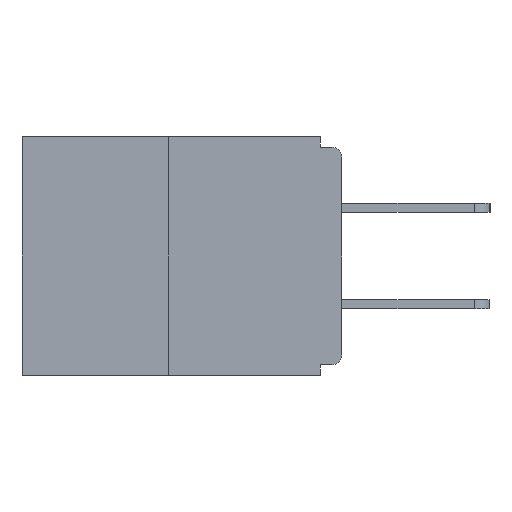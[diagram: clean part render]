
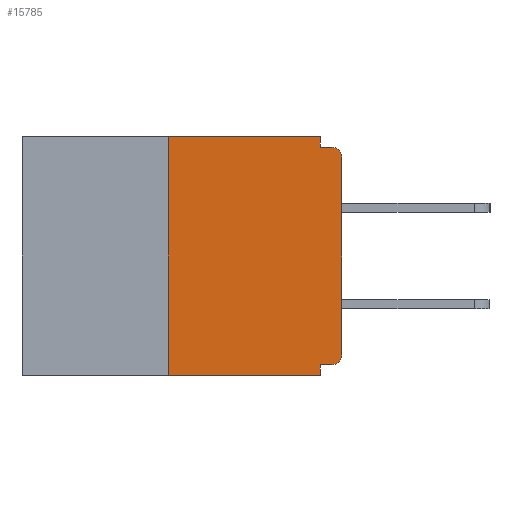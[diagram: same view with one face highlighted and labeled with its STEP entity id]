
A CAD part, left-side view. The second image highlights one B-rep face of the part: STEP entity #15785.
In plain terms, the highlighted planar face has unit normal (-1, 0, 0).
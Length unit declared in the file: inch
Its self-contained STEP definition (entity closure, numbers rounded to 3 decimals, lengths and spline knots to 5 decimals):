
#583 = VERTEX_POINT ( 'NONE', #587 ) ;
#587 = CARTESIAN_POINT ( 'NONE',  ( 0., 0.25, -0.343 ) ) ;
#1026 = ORIENTED_EDGE ( 'NONE', *, *, #21124, .T. ) ;
#1037 = VERTEX_POINT ( 'NONE', #14218 ) ;
#1105 = VECTOR ( 'NONE', #7954, 39.37008 ) ;
#1210 = CARTESIAN_POINT ( 'NONE',  ( 0., 0.031, 0. ) ) ;
#1218 = LINE ( 'NONE', #15127, #15951 ) ;
#1472 = VERTEX_POINT ( 'NONE', #10918 ) ;
#2548 = EDGE_CURVE ( 'NONE', #1472, #4662, #10265, .T. ) ;
#2583 = EDGE_CURVE ( 'NONE', #6001, #6195, #3032, .T. ) ;
#2666 = DIRECTION ( 'NONE',  ( -1., 0., 0. ) ) ;
#2923 = DIRECTION ( 'NONE',  ( 0., 0., -1. ) ) ;
#2991 = DIRECTION ( 'NONE',  ( 0., 1., 0. ) ) ;
#3032 = LINE ( 'NONE', #17066, #6735 ) ;
#3038 = CARTESIAN_POINT ( 'NONE',  ( 0., 0.031, -0.343 ) ) ;
#3102 = CARTESIAN_POINT ( 'NONE',  ( 0., 0.015, -0.313 ) ) ;
#3447 = ORIENTED_EDGE ( 'NONE', *, *, #2548, .F. ) ;
#3737 = DIRECTION ( 'NONE',  ( 0., 0., 1. ) ) ;
#3968 = VECTOR ( 'NONE', #3737, 39.37008 ) ;
#4325 = ORIENTED_EDGE ( 'NONE', *, *, #5845, .T. ) ;
#4597 = EDGE_CURVE ( 'NONE', #583, #5198, #10309, .T. ) ;
#4662 = VERTEX_POINT ( 'NONE', #20877 ) ;
#4732 = LINE ( 'NONE', #3038, #16890 ) ;
#5198 = VERTEX_POINT ( 'NONE', #12445 ) ;
#5516 = CIRCLE ( 'NONE', #6627, 0.015 ) ;
#5822 = CIRCLE ( 'NONE', #8770, 0.015 ) ;
#5845 = EDGE_CURVE ( 'NONE', #8885, #6001, #5822, .T. ) ;
#5857 = FACE_OUTER_BOUND ( 'NONE', #8430, .T. ) ;
#6001 = VERTEX_POINT ( 'NONE', #12613 ) ;
#6045 = EDGE_CURVE ( 'NONE', #20581, #1472, #10163, .T. ) ;
#6168 = EDGE_CURVE ( 'NONE', #1037, #21715, #4732, .T. ) ;
#6195 = VERTEX_POINT ( 'NONE', #10719 ) ;
#6202 = CARTESIAN_POINT ( 'NONE',  ( 0., 0.015, -0.03 ) ) ;
#6627 = AXIS2_PLACEMENT_3D ( 'NONE', #6202, #2666, #17145 ) ;
#6629 = DIRECTION ( 'NONE',  ( 0., 0., -1. ) ) ;
#6664 = AXIS2_PLACEMENT_3D ( 'NONE', #20034, #12877, #18069 ) ;
#6682 = CARTESIAN_POINT ( 'NONE',  ( 0., 0., -0.015 ) ) ;
#6735 = VECTOR ( 'NONE', #20732, 39.37008 ) ;
#7196 = ORIENTED_EDGE ( 'NONE', *, *, #9436, .T. ) ;
#7348 = ORIENTED_EDGE ( 'NONE', *, *, #20158, .F. ) ;
#7954 = DIRECTION ( 'NONE',  ( 0., 0., -1. ) ) ;
#8401 = DIRECTION ( 'NONE',  ( 0., -1., 0. ) ) ;
#8430 = EDGE_LOOP ( 'NONE', ( #17635, #21304, #1026, #21549, #7348, #4325, #9006, #7196, #3447, #8895 ) ) ;
#8770 = AXIS2_PLACEMENT_3D ( 'NONE', #3102, #15724, #6629 ) ;
#8885 = VERTEX_POINT ( 'NONE', #16389 ) ;
#8895 = ORIENTED_EDGE ( 'NONE', *, *, #6045, .F. ) ;
#9006 = ORIENTED_EDGE ( 'NONE', *, *, #2583, .T. ) ;
#9436 = EDGE_CURVE ( 'NONE', #6195, #4662, #5516, .T. ) ;
#10163 = LINE ( 'NONE', #1210, #1105 ) ;
#10265 = LINE ( 'NONE', #6682, #17406 ) ;
#10309 = LINE ( 'NONE', #15948, #3968 ) ;
#10536 = CARTESIAN_POINT ( 'NONE',  ( 0., 0.031, 0. ) ) ;
#10719 = CARTESIAN_POINT ( 'NONE',  ( 0., 0., -0.03 ) ) ;
#10918 = CARTESIAN_POINT ( 'NONE',  ( 0., 0.031, -0.015 ) ) ;
#11724 = CARTESIAN_POINT ( 'NONE',  ( 0., 0., -0.328 ) ) ;
#11834 = LINE ( 'NONE', #11724, #13751 ) ;
#12445 = CARTESIAN_POINT ( 'NONE',  ( 0., 0.25, 0. ) ) ;
#12613 = CARTESIAN_POINT ( 'NONE',  ( 0., 0., -0.313 ) ) ;
#12877 = DIRECTION ( 'NONE',  ( 1., 0., 0. ) ) ;
#13751 = VECTOR ( 'NONE', #2991, 39.37008 ) ;
#14218 = CARTESIAN_POINT ( 'NONE',  ( 0., 0.031, -0.328 ) ) ;
#14423 = CARTESIAN_POINT ( 'NONE',  ( 0., 0.46, -0.343 ) ) ;
#15127 = CARTESIAN_POINT ( 'NONE',  ( 0., 0.46, 0. ) ) ;
#15724 = DIRECTION ( 'NONE',  ( -1., 0., 0. ) ) ;
#15785 = ADVANCED_FACE ( 'NONE', ( #5857 ), #19686, .F. ) ;
#15948 = CARTESIAN_POINT ( 'NONE',  ( 0., 0.25, 0. ) ) ;
#15951 = VECTOR ( 'NONE', #18666, 39.37008 ) ;
#16256 = LINE ( 'NONE', #14423, #20763 ) ;
#16389 = CARTESIAN_POINT ( 'NONE',  ( 0., 0.015, -0.328 ) ) ;
#16786 = CARTESIAN_POINT ( 'NONE',  ( 0., 0.031, -0.343 ) ) ;
#16890 = VECTOR ( 'NONE', #2923, 39.37008 ) ;
#17066 = CARTESIAN_POINT ( 'NONE',  ( 0., 0., 0. ) ) ;
#17145 = DIRECTION ( 'NONE',  ( 0., 0., -1. ) ) ;
#17406 = VECTOR ( 'NONE', #8401, 39.37008 ) ;
#17635 = ORIENTED_EDGE ( 'NONE', *, *, #19852, .F. ) ;
#17760 = DIRECTION ( 'NONE',  ( 0., -1., 0. ) ) ;
#18069 = DIRECTION ( 'NONE',  ( 0., 0., -1. ) ) ;
#18666 = DIRECTION ( 'NONE',  ( 0., -1., 0. ) ) ;
#19686 = PLANE ( 'NONE',  #6664 ) ;
#19852 = EDGE_CURVE ( 'NONE', #5198, #20581, #1218, .T. ) ;
#20034 = CARTESIAN_POINT ( 'NONE',  ( 0., 0.46, 0. ) ) ;
#20158 = EDGE_CURVE ( 'NONE', #8885, #1037, #11834, .T. ) ;
#20581 = VERTEX_POINT ( 'NONE', #10536 ) ;
#20732 = DIRECTION ( 'NONE',  ( 0., 0., 1. ) ) ;
#20763 = VECTOR ( 'NONE', #17760, 39.37008 ) ;
#20877 = CARTESIAN_POINT ( 'NONE',  ( 0., 0.015, -0.015 ) ) ;
#21124 = EDGE_CURVE ( 'NONE', #583, #21715, #16256, .T. ) ;
#21304 = ORIENTED_EDGE ( 'NONE', *, *, #4597, .F. ) ;
#21549 = ORIENTED_EDGE ( 'NONE', *, *, #6168, .F. ) ;
#21715 = VERTEX_POINT ( 'NONE', #16786 ) ;
